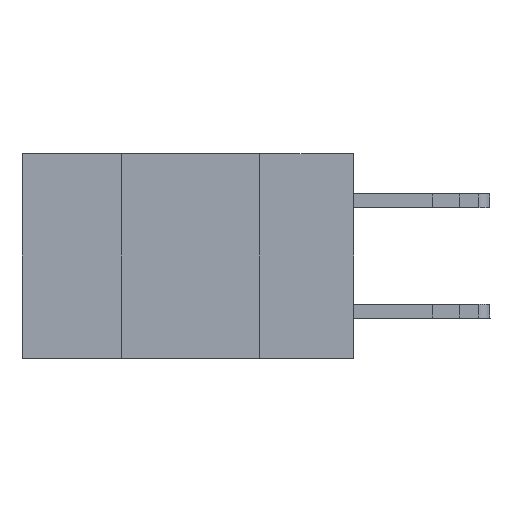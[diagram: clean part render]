
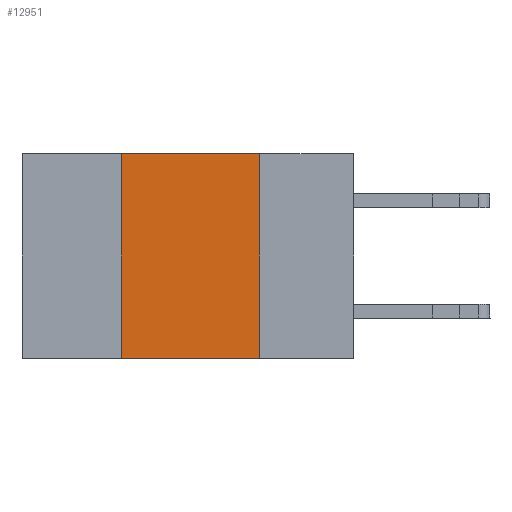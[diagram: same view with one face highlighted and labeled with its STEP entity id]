
A CAD part, left-side view. The second image highlights one B-rep face of the part: STEP entity #12951.
In plain terms, the highlighted planar face has unit normal (-1, 0, 0).
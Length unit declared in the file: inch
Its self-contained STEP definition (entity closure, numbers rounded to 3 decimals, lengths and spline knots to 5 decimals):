
#383 = VECTOR ( 'NONE', #2458, 39.37008 ) ;
#500 = CARTESIAN_POINT ( 'NONE',  ( 0., 0.42, -0.37 ) ) ;
#758 = DIRECTION ( 'NONE',  ( 0., 0., -1. ) ) ;
#1034 = VERTEX_POINT ( 'NONE', #500 ) ;
#1360 = VERTEX_POINT ( 'NONE', #16139 ) ;
#2245 = ORIENTED_EDGE ( 'NONE', *, *, #8309, .F. ) ;
#2452 = ORIENTED_EDGE ( 'NONE', *, *, #7543, .T. ) ;
#2458 = DIRECTION ( 'NONE',  ( 0., -1., 0. ) ) ;
#2667 = ORIENTED_EDGE ( 'NONE', *, *, #6233, .F. ) ;
#3013 = ORIENTED_EDGE ( 'NONE', *, *, #3837, .F. ) ;
#3496 = LINE ( 'NONE', #5619, #18738 ) ;
#3721 = CARTESIAN_POINT ( 'NONE',  ( 0., 0.17, 0. ) ) ;
#3828 = EDGE_LOOP ( 'NONE', ( #2667, #3013, #2245, #2452 ) ) ;
#3837 = EDGE_CURVE ( 'NONE', #6311, #4466, #15788, .T. ) ;
#4466 = VERTEX_POINT ( 'NONE', #9861 ) ;
#5208 = DIRECTION ( 'NONE',  ( 0., 0., -1. ) ) ;
#5251 = CARTESIAN_POINT ( 'NONE',  ( 0., 0.6, -0.37 ) ) ;
#5276 = PLANE ( 'NONE',  #16989 ) ;
#5619 = CARTESIAN_POINT ( 'NONE',  ( 0., 0.42, 0. ) ) ;
#6233 = EDGE_CURVE ( 'NONE', #4466, #1360, #6954, .T. ) ;
#6311 = VERTEX_POINT ( 'NONE', #6938 ) ;
#6787 = DIRECTION ( 'NONE',  ( 0., -1., 0. ) ) ;
#6938 = CARTESIAN_POINT ( 'NONE',  ( 0., 0.42, 0. ) ) ;
#6954 = LINE ( 'NONE', #3721, #14342 ) ;
#7543 = EDGE_CURVE ( 'NONE', #1034, #1360, #9150, .T. ) ;
#8309 = EDGE_CURVE ( 'NONE', #1034, #6311, #3496, .T. ) ;
#8311 = CARTESIAN_POINT ( 'NONE',  ( 0., 0.6, 0. ) ) ;
#9150 = LINE ( 'NONE', #5251, #16489 ) ;
#9797 = DIRECTION ( 'NONE',  ( 1., 0., 0. ) ) ;
#9861 = CARTESIAN_POINT ( 'NONE',  ( 0., 0.17, 0. ) ) ;
#10126 = DIRECTION ( 'NONE',  ( 0., 0., 1. ) ) ;
#10316 = FACE_OUTER_BOUND ( 'NONE', #3828, .T. ) ;
#12951 = ADVANCED_FACE ( 'NONE', ( #10316 ), #5276, .F. ) ;
#14342 = VECTOR ( 'NONE', #5208, 39.37008 ) ;
#15788 = LINE ( 'NONE', #17279, #383 ) ;
#16139 = CARTESIAN_POINT ( 'NONE',  ( 0., 0.17, -0.37 ) ) ;
#16489 = VECTOR ( 'NONE', #6787, 39.37008 ) ;
#16989 = AXIS2_PLACEMENT_3D ( 'NONE', #8311, #9797, #758 ) ;
#17279 = CARTESIAN_POINT ( 'NONE',  ( 0., 0.6, 0. ) ) ;
#18738 = VECTOR ( 'NONE', #10126, 39.37008 ) ;
